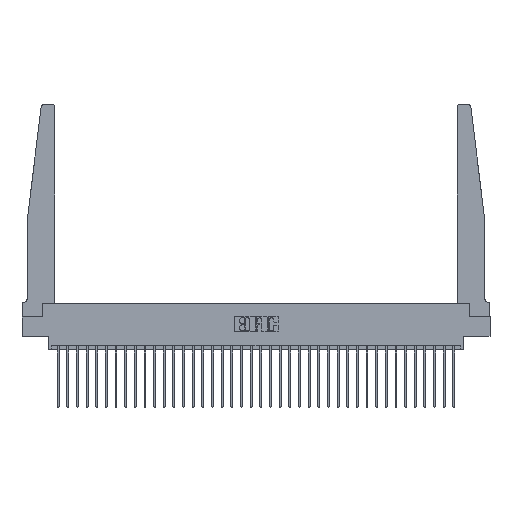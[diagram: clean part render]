
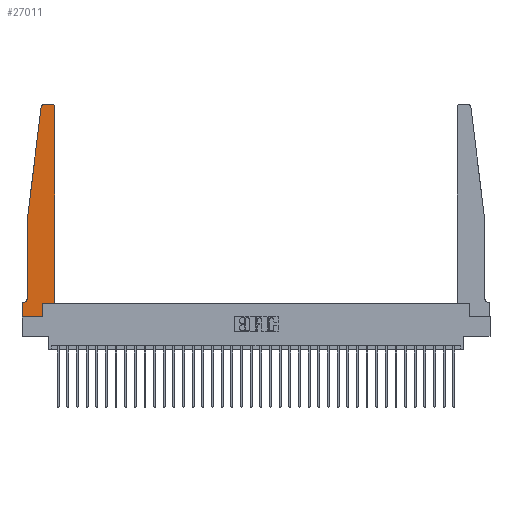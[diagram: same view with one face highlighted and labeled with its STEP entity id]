
A CAD part, top view. The second image highlights one B-rep face of the part: STEP entity #27011.
In plain terms, the highlighted planar face has unit normal (0, 0, 1).
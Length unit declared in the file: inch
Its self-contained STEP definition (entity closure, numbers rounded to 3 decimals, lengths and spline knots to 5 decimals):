
#494 = DIRECTION ( 'NONE',  ( 1., 0., 0. ) ) ;
#821 = VERTEX_POINT ( 'NONE', #4563 ) ;
#855 = AXIS2_PLACEMENT_3D ( 'NONE', #20556, #27882, #494 ) ;
#970 = EDGE_CURVE ( 'NONE', #821, #20450, #30441, .T. ) ;
#1367 = DIRECTION ( 'NONE',  ( 1., 0., 0. ) ) ;
#1533 = CARTESIAN_POINT ( 'NONE',  ( 0.425, 0.18, 0.37 ) ) ;
#1695 = CARTESIAN_POINT ( 'NONE',  ( 0., 0., 0.37 ) ) ;
#2282 = CARTESIAN_POINT ( 'NONE',  ( 0.2605, 0.18, 0.37 ) ) ;
#3263 = ORIENTED_EDGE ( 'NONE', *, *, #29117, .T. ) ;
#3366 = DIRECTION ( 'NONE',  ( 0., 0., 1. ) ) ;
#3880 = CARTESIAN_POINT ( 'NONE',  ( 0.425, 0.18, 0.37 ) ) ;
#4138 = VECTOR ( 'NONE', #20275, 39.37008 ) ;
#4145 = LINE ( 'NONE', #14095, #18272 ) ;
#4243 = CARTESIAN_POINT ( 'NONE',  ( 0.065, 1.25, 0.37 ) ) ;
#4454 = VERTEX_POINT ( 'NONE', #14684 ) ;
#4563 = CARTESIAN_POINT ( 'NONE',  ( 0.015, 0.1875, 0.37 ) ) ;
#4875 = CARTESIAN_POINT ( 'NONE',  ( 0., 0., 0.37 ) ) ;
#4890 = ORIENTED_EDGE ( 'NONE', *, *, #22601, .T. ) ;
#5498 = VECTOR ( 'NONE', #27005, 39.37008 ) ;
#5625 = EDGE_CURVE ( 'NONE', #28890, #22166, #16842, .T. ) ;
#5846 = CARTESIAN_POINT ( 'NONE',  ( 0.395, 2.72, 0.37 ) ) ;
#5900 = ORIENTED_EDGE ( 'NONE', *, *, #32123, .T. ) ;
#5968 = DIRECTION ( 'NONE',  ( 0., 0., 1. ) ) ;
#6284 = CARTESIAN_POINT ( 'NONE',  ( 0.425, 2.72, 0.37 ) ) ;
#6781 = CIRCLE ( 'NONE', #15265, 0.03 ) ;
#7216 = CIRCLE ( 'NONE', #24678, 0.03 ) ;
#7374 = CARTESIAN_POINT ( 'NONE',  ( 0.425, 0.18, 0.37 ) ) ;
#7614 = CARTESIAN_POINT ( 'NONE',  ( 0.27653, 2.75, 0.37 ) ) ;
#7857 = EDGE_CURVE ( 'NONE', #9964, #32269, #4145, .T. ) ;
#8478 = DIRECTION ( 'NONE',  ( 0., 0., -1. ) ) ;
#9266 = ORIENTED_EDGE ( 'NONE', *, *, #21782, .T. ) ;
#9765 = CARTESIAN_POINT ( 'NONE',  ( 0.2605, 0.18, 0.37 ) ) ;
#9964 = VERTEX_POINT ( 'NONE', #20642 ) ;
#10028 = DIRECTION ( 'NONE',  ( -1., 0., 0. ) ) ;
#10459 = PLANE ( 'NONE',  #855 ) ;
#10549 = EDGE_CURVE ( 'NONE', #22166, #4454, #16311, .T. ) ;
#10663 = LINE ( 'NONE', #7374, #4138 ) ;
#10973 = ORIENTED_EDGE ( 'NONE', *, *, #29025, .T. ) ;
#11842 = CARTESIAN_POINT ( 'NONE',  ( 0., 0.1875, 0.37 ) ) ;
#11956 = VERTEX_POINT ( 'NONE', #6284 ) ;
#11967 = ORIENTED_EDGE ( 'NONE', *, *, #970, .T. ) ;
#12178 = LINE ( 'NONE', #4875, #21343 ) ;
#12953 = FACE_OUTER_BOUND ( 'NONE', #13603, .T. ) ;
#12959 = EDGE_CURVE ( 'NONE', #15715, #29303, #18795, .T. ) ;
#13603 = EDGE_LOOP ( 'NONE', ( #27407, #24380, #20192, #22791, #5900, #11967, #24998, #9266, #4890, #30645, #10973, #3263 ) ) ;
#14095 = CARTESIAN_POINT ( 'NONE',  ( 0.25, 2.75, 0.37 ) ) ;
#14358 = DIRECTION ( 'NONE',  ( -0.122, -0.992, 0. ) ) ;
#14684 = CARTESIAN_POINT ( 'NONE',  ( 0.065, 0.2375, 0.37 ) ) ;
#15000 = CARTESIAN_POINT ( 'NONE',  ( 0.24675, 2.72367, 0.37 ) ) ;
#15265 = AXIS2_PLACEMENT_3D ( 'NONE', #5846, #3366, #1367 ) ;
#15715 = VERTEX_POINT ( 'NONE', #2282 ) ;
#15816 = DIRECTION ( 'NONE',  ( 0., -1., 0. ) ) ;
#16261 = DIRECTION ( 'NONE',  ( 1., 0., 0. ) ) ;
#16311 = LINE ( 'NONE', #18457, #32182 ) ;
#16421 = DIRECTION ( 'NONE',  ( -1., 0., 0. ) ) ;
#16842 = LINE ( 'NONE', #4243, #28857 ) ;
#17444 = EDGE_CURVE ( 'NONE', #20450, #26750, #32601, .T. ) ;
#17493 = DIRECTION ( 'NONE',  ( 0., -1., 0. ) ) ;
#18088 = VERTEX_POINT ( 'NONE', #20409 ) ;
#18272 = VECTOR ( 'NONE', #16421, 39.37008 ) ;
#18457 = CARTESIAN_POINT ( 'NONE',  ( 0.065, 1.25, 0.37 ) ) ;
#18739 = DIRECTION ( 'NONE',  ( -1., 0., 0. ) ) ;
#18795 = LINE ( 'NONE', #3880, #21672 ) ;
#19970 = CARTESIAN_POINT ( 'NONE',  ( 0., 0., 0.37 ) ) ;
#20095 = CIRCLE ( 'NONE', #27511, 0.05 ) ;
#20192 = ORIENTED_EDGE ( 'NONE', *, *, #5625, .T. ) ;
#20275 = DIRECTION ( 'NONE',  ( 0., 1., 0. ) ) ;
#20409 = CARTESIAN_POINT ( 'NONE',  ( 0.2605, 0., 0.37 ) ) ;
#20450 = VERTEX_POINT ( 'NONE', #11842 ) ;
#20556 = CARTESIAN_POINT ( 'NONE',  ( 0., 0.1875, 0.37 ) ) ;
#20642 = CARTESIAN_POINT ( 'NONE',  ( 0.395, 2.75, 0.37 ) ) ;
#21343 = VECTOR ( 'NONE', #22262, 39.37008 ) ;
#21672 = VECTOR ( 'NONE', #21760, 39.37008 ) ;
#21760 = DIRECTION ( 'NONE',  ( 1., 0., 0. ) ) ;
#21782 = EDGE_CURVE ( 'NONE', #26750, #18088, #12178, .T. ) ;
#22083 = VECTOR ( 'NONE', #10028, 39.37008 ) ;
#22166 = VERTEX_POINT ( 'NONE', #32053 ) ;
#22262 = DIRECTION ( 'NONE',  ( 1., 0., 0. ) ) ;
#22601 = EDGE_CURVE ( 'NONE', #18088, #15715, #24854, .T. ) ;
#22791 = ORIENTED_EDGE ( 'NONE', *, *, #10549, .T. ) ;
#24380 = ORIENTED_EDGE ( 'NONE', *, *, #27098, .T. ) ;
#24678 = AXIS2_PLACEMENT_3D ( 'NONE', #26694, #5968, #16261 ) ;
#24854 = LINE ( 'NONE', #9765, #5498 ) ;
#24998 = ORIENTED_EDGE ( 'NONE', *, *, #17444, .T. ) ;
#26694 = CARTESIAN_POINT ( 'NONE',  ( 0.27653, 2.72, 0.37 ) ) ;
#26750 = VERTEX_POINT ( 'NONE', #1695 ) ;
#27005 = DIRECTION ( 'NONE',  ( 0., 1., 0. ) ) ;
#27011 = ADVANCED_FACE ( 'NONE', ( #12953 ), #10459, .T. ) ;
#27098 = EDGE_CURVE ( 'NONE', #32269, #28890, #7216, .T. ) ;
#27100 = VECTOR ( 'NONE', #17493, 39.37008 ) ;
#27407 = ORIENTED_EDGE ( 'NONE', *, *, #7857, .T. ) ;
#27511 = AXIS2_PLACEMENT_3D ( 'NONE', #31051, #8478, #18739 ) ;
#27882 = DIRECTION ( 'NONE',  ( 0., 0., 1. ) ) ;
#28857 = VECTOR ( 'NONE', #14358, 39.37008 ) ;
#28890 = VERTEX_POINT ( 'NONE', #15000 ) ;
#29025 = EDGE_CURVE ( 'NONE', #29303, #11956, #10663, .T. ) ;
#29117 = EDGE_CURVE ( 'NONE', #11956, #9964, #6781, .T. ) ;
#29303 = VERTEX_POINT ( 'NONE', #1533 ) ;
#30273 = CARTESIAN_POINT ( 'NONE',  ( 0.065, 0.1875, 0.37 ) ) ;
#30441 = LINE ( 'NONE', #30273, #22083 ) ;
#30645 = ORIENTED_EDGE ( 'NONE', *, *, #12959, .T. ) ;
#31051 = CARTESIAN_POINT ( 'NONE',  ( 0.015, 0.2375, 0.37 ) ) ;
#32053 = CARTESIAN_POINT ( 'NONE',  ( 0.065, 1.25, 0.37 ) ) ;
#32123 = EDGE_CURVE ( 'NONE', #4454, #821, #20095, .T. ) ;
#32182 = VECTOR ( 'NONE', #15816, 39.37008 ) ;
#32269 = VERTEX_POINT ( 'NONE', #7614 ) ;
#32601 = LINE ( 'NONE', #19970, #27100 ) ;
